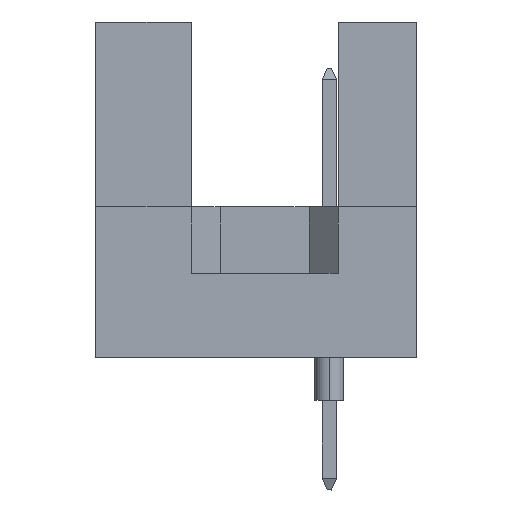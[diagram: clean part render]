
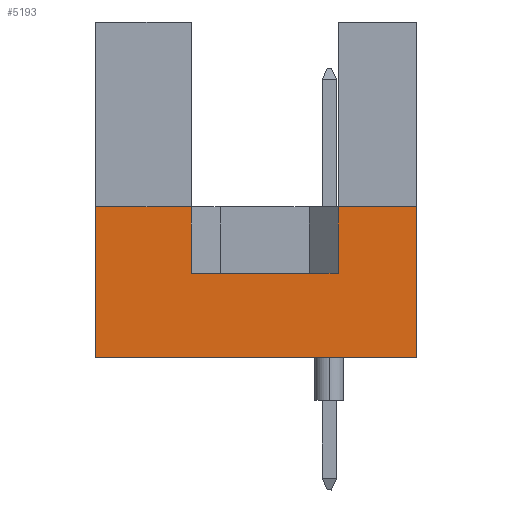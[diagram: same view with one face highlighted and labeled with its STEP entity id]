
A CAD part, left-side view. The second image highlights one B-rep face of the part: STEP entity #5193.
In plain terms, the highlighted planar face has unit normal (-1, 0, 0).
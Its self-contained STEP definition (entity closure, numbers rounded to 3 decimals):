
#219 = CARTESIAN_POINT ( 'NONE',  ( -47.5, 11.1, 5.2 ) ) ;
#754 = VERTEX_POINT ( 'NONE', #11140 ) ;
#1028 = CARTESIAN_POINT ( 'NONE',  ( -47.5, 2.71, 2.9 ) ) ;
#1714 = CARTESIAN_POINT ( 'NONE',  ( -47.5, 2.71, 5.2 ) ) ;
#2047 = EDGE_CURVE ( 'NONE', #8260, #3152, #8664, .T. ) ;
#2187 = EDGE_CURVE ( 'NONE', #14998, #16327, #16549, .T. ) ;
#2517 = ORIENTED_EDGE ( 'NONE', *, *, #6977, .T. ) ;
#2942 = VERTEX_POINT ( 'NONE', #8633 ) ;
#2977 = CARTESIAN_POINT ( 'NONE',  ( -47.5, 7.79, 2.9 ) ) ;
#3152 = VERTEX_POINT ( 'NONE', #1714 ) ;
#3305 = DIRECTION ( 'NONE',  ( 0., -1., 0. ) ) ;
#4549 = FACE_OUTER_BOUND ( 'NONE', #15238, .T. ) ;
#4919 = LINE ( 'NONE', #8635, #11100 ) ;
#5114 = CARTESIAN_POINT ( 'NONE',  ( -47.5, 0., 0. ) ) ;
#5129 = LINE ( 'NONE', #10253, #8523 ) ;
#5193 = ADVANCED_FACE ( 'NONE', ( #4549 ), #8593, .F. ) ;
#5430 = EDGE_CURVE ( 'NONE', #8021, #2942, #13188, .T. ) ;
#5813 = VECTOR ( 'NONE', #6465, 1000. ) ;
#6465 = DIRECTION ( 'NONE',  ( 0., 0., 1. ) ) ;
#6543 = VERTEX_POINT ( 'NONE', #15920 ) ;
#6796 = DIRECTION ( 'NONE',  ( 0., -1., 0. ) ) ;
#6977 = EDGE_CURVE ( 'NONE', #754, #14998, #9689, .T. ) ;
#7245 = DIRECTION ( 'NONE',  ( 0., 0., -1. ) ) ;
#7422 = CARTESIAN_POINT ( 'NONE',  ( -47.5, 0., 0. ) ) ;
#7556 = DIRECTION ( 'NONE',  ( 0., 0., 1. ) ) ;
#8021 = VERTEX_POINT ( 'NONE', #219 ) ;
#8026 = LINE ( 'NONE', #2977, #11509 ) ;
#8073 = EDGE_CURVE ( 'NONE', #6543, #2942, #8026, .T. ) ;
#8249 = DIRECTION ( 'NONE',  ( 1., 0., 0. ) ) ;
#8260 = VERTEX_POINT ( 'NONE', #9860 ) ;
#8523 = VECTOR ( 'NONE', #15622, 1000. ) ;
#8593 = PLANE ( 'NONE',  #13768 ) ;
#8633 = CARTESIAN_POINT ( 'NONE',  ( -47.5, 7.79, 5.2 ) ) ;
#8635 = CARTESIAN_POINT ( 'NONE',  ( -47.5, 7.79, 2.9 ) ) ;
#8664 = LINE ( 'NONE', #1028, #15477 ) ;
#9401 = CARTESIAN_POINT ( 'NONE',  ( -47.5, 11.1, 5.2 ) ) ;
#9445 = EDGE_CURVE ( 'NONE', #6543, #8260, #4919, .T. ) ;
#9689 = LINE ( 'NONE', #14630, #13147 ) ;
#9859 = ORIENTED_EDGE ( 'NONE', *, *, #9445, .F. ) ;
#9860 = CARTESIAN_POINT ( 'NONE',  ( -47.5, 2.71, 2.9 ) ) ;
#9995 = DIRECTION ( 'NONE',  ( 0., 0., 1. ) ) ;
#10253 = CARTESIAN_POINT ( 'NONE',  ( -47.5, 11.1, 5.2 ) ) ;
#10951 = ORIENTED_EDGE ( 'NONE', *, *, #12691, .F. ) ;
#11092 = ORIENTED_EDGE ( 'NONE', *, *, #2187, .T. ) ;
#11100 = VECTOR ( 'NONE', #13823, 1000. ) ;
#11140 = CARTESIAN_POINT ( 'NONE',  ( -47.5, 11.1, 0. ) ) ;
#11437 = ORIENTED_EDGE ( 'NONE', *, *, #2047, .F. ) ;
#11505 = CARTESIAN_POINT ( 'NONE',  ( -47.5, 11.1, 0. ) ) ;
#11509 = VECTOR ( 'NONE', #15577, 1000. ) ;
#12509 = LINE ( 'NONE', #11505, #12773 ) ;
#12691 = EDGE_CURVE ( 'NONE', #754, #8021, #12509, .T. ) ;
#12773 = VECTOR ( 'NONE', #7556, 1000. ) ;
#12990 = ORIENTED_EDGE ( 'NONE', *, *, #8073, .T. ) ;
#13147 = VECTOR ( 'NONE', #3305, 1000. ) ;
#13188 = LINE ( 'NONE', #9401, #14580 ) ;
#13708 = CARTESIAN_POINT ( 'NONE',  ( -47.5, 11.1, 0. ) ) ;
#13768 = AXIS2_PLACEMENT_3D ( 'NONE', #13708, #8249, #7245 ) ;
#13823 = DIRECTION ( 'NONE',  ( 0., -1., 0. ) ) ;
#13846 = EDGE_CURVE ( 'NONE', #3152, #16327, #5129, .T. ) ;
#14082 = ORIENTED_EDGE ( 'NONE', *, *, #5430, .F. ) ;
#14555 = ORIENTED_EDGE ( 'NONE', *, *, #13846, .F. ) ;
#14580 = VECTOR ( 'NONE', #6796, 1000. ) ;
#14630 = CARTESIAN_POINT ( 'NONE',  ( -47.5, 11.1, 0. ) ) ;
#14998 = VERTEX_POINT ( 'NONE', #7422 ) ;
#15238 = EDGE_LOOP ( 'NONE', ( #9859, #12990, #14082, #10951, #2517, #11092, #14555, #11437 ) ) ;
#15477 = VECTOR ( 'NONE', #9995, 1000. ) ;
#15577 = DIRECTION ( 'NONE',  ( 0., 0., 1. ) ) ;
#15622 = DIRECTION ( 'NONE',  ( 0., -1., 0. ) ) ;
#15920 = CARTESIAN_POINT ( 'NONE',  ( -47.5, 7.79, 2.9 ) ) ;
#16327 = VERTEX_POINT ( 'NONE', #16331 ) ;
#16331 = CARTESIAN_POINT ( 'NONE',  ( -47.5, 0., 5.2 ) ) ;
#16549 = LINE ( 'NONE', #5114, #5813 ) ;
